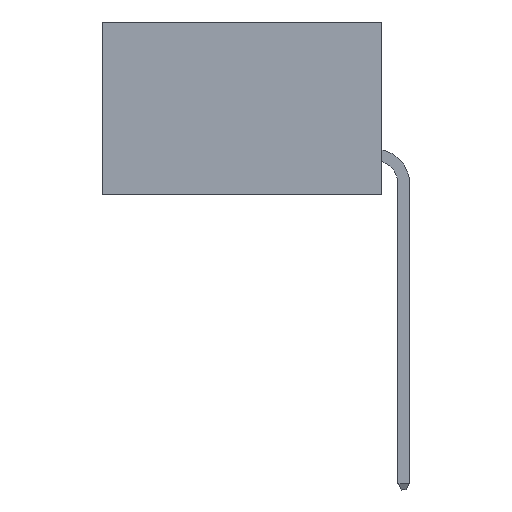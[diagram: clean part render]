
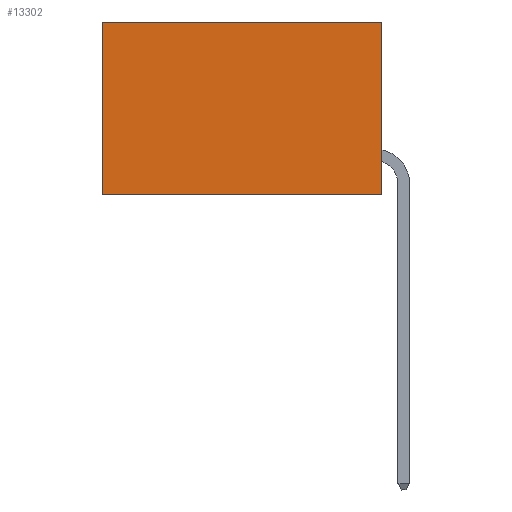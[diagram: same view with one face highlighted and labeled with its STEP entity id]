
A CAD part, left-side view. The second image highlights one B-rep face of the part: STEP entity #13302.
In plain terms, the highlighted planar face has unit normal (-1, 0, 0).
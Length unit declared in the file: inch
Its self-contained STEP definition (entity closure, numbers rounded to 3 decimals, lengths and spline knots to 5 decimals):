
#280 = EDGE_CURVE ( 'NONE', #14151, #20605, #5463, .T. ) ;
#896 = CARTESIAN_POINT ( 'NONE',  ( 0.2875, 0.6, 0. ) ) ;
#1261 = PLANE ( 'NONE',  #11829 ) ;
#1429 = FACE_OUTER_BOUND ( 'NONE', #25678, .T. ) ;
#2150 = VERTEX_POINT ( 'NONE', #7316 ) ;
#3501 = DIRECTION ( 'NONE',  ( 0., 0., -1. ) ) ;
#4729 = DIRECTION ( 'NONE',  ( 0., 1., 0. ) ) ;
#5463 = LINE ( 'NONE', #13765, #22353 ) ;
#5796 = CARTESIAN_POINT ( 'NONE',  ( 0.2875, 0., 0. ) ) ;
#7316 = CARTESIAN_POINT ( 'NONE',  ( 0.2875, 0.6, -0.37 ) ) ;
#7693 = EDGE_CURVE ( 'NONE', #14151, #15286, #17287, .T. ) ;
#7852 = ORIENTED_EDGE ( 'NONE', *, *, #17798, .F. ) ;
#7962 = DIRECTION ( 'NONE',  ( 0., 1., 0. ) ) ;
#9834 = DIRECTION ( 'NONE',  ( 0., 0., -1. ) ) ;
#11201 = LINE ( 'NONE', #896, #16867 ) ;
#11829 = AXIS2_PLACEMENT_3D ( 'NONE', #20432, #16354, #3501 ) ;
#11947 = CARTESIAN_POINT ( 'NONE',  ( 0.2875, 0.6, 0. ) ) ;
#13302 = ADVANCED_FACE ( 'NONE', ( #1429 ), #1261, .F. ) ;
#13765 = CARTESIAN_POINT ( 'NONE',  ( 0.2875, 0., 0. ) ) ;
#14151 = VERTEX_POINT ( 'NONE', #22659 ) ;
#14716 = ORIENTED_EDGE ( 'NONE', *, *, #280, .F. ) ;
#15286 = VERTEX_POINT ( 'NONE', #11947 ) ;
#16354 = DIRECTION ( 'NONE',  ( 1., 0., 0. ) ) ;
#16867 = VECTOR ( 'NONE', #26596, 39.37008 ) ;
#17287 = LINE ( 'NONE', #5796, #23524 ) ;
#17798 = EDGE_CURVE ( 'NONE', #20605, #2150, #27194, .T. ) ;
#19029 = ORIENTED_EDGE ( 'NONE', *, *, #22510, .T. ) ;
#20432 = CARTESIAN_POINT ( 'NONE',  ( 0.2875, 0., 0. ) ) ;
#20605 = VERTEX_POINT ( 'NONE', #24652 ) ;
#21525 = VECTOR ( 'NONE', #4729, 39.37008 ) ;
#21602 = CARTESIAN_POINT ( 'NONE',  ( 0.2875, 0., -0.37 ) ) ;
#21766 = ORIENTED_EDGE ( 'NONE', *, *, #7693, .T. ) ;
#22353 = VECTOR ( 'NONE', #9834, 39.37008 ) ;
#22510 = EDGE_CURVE ( 'NONE', #15286, #2150, #11201, .T. ) ;
#22659 = CARTESIAN_POINT ( 'NONE',  ( 0.2875, 0., 0. ) ) ;
#23524 = VECTOR ( 'NONE', #7962, 39.37008 ) ;
#24652 = CARTESIAN_POINT ( 'NONE',  ( 0.2875, 0., -0.37 ) ) ;
#25678 = EDGE_LOOP ( 'NONE', ( #19029, #7852, #14716, #21766 ) ) ;
#26596 = DIRECTION ( 'NONE',  ( 0., 0., -1. ) ) ;
#27194 = LINE ( 'NONE', #21602, #21525 ) ;
